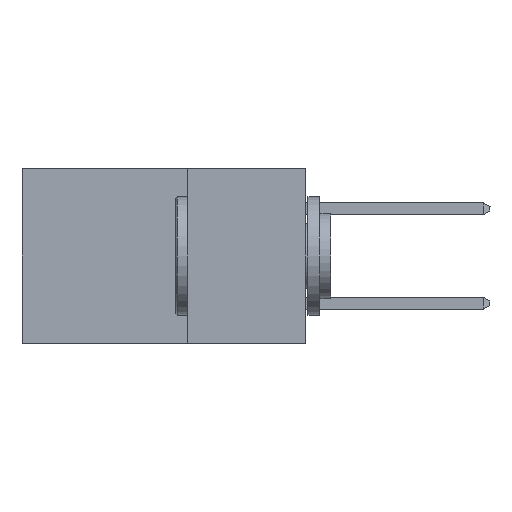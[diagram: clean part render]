
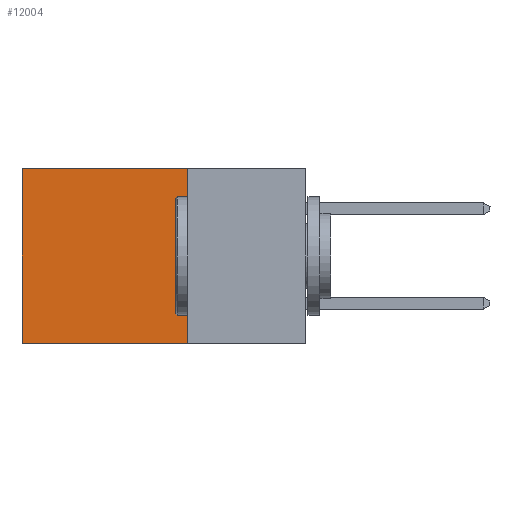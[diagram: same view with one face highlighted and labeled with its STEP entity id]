
A CAD part, left-side view. The second image highlights one B-rep face of the part: STEP entity #12004.
In plain terms, the highlighted planar face has unit normal (-1, 0, 0).
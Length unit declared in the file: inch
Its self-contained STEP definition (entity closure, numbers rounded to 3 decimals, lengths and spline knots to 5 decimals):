
#1661 = AXIS2_PLACEMENT_3D ( 'NONE', #18936, #21601, #6206 ) ;
#2513 = EDGE_CURVE ( 'NONE', #15147, #22574, #18310, .T. ) ;
#3587 = PLANE ( 'NONE',  #1661 ) ;
#4843 = EDGE_LOOP ( 'NONE', ( #19718, #20864, #5528, #10257 ) ) ;
#5085 = CARTESIAN_POINT ( 'NONE',  ( 0.298, 0.25, 0. ) ) ;
#5528 = ORIENTED_EDGE ( 'NONE', *, *, #19236, .F. ) ;
#5930 = LINE ( 'NONE', #11787, #24842 ) ;
#6206 = DIRECTION ( 'NONE',  ( 0., 0., -1. ) ) ;
#6386 = VERTEX_POINT ( 'NONE', #13751 ) ;
#10257 = ORIENTED_EDGE ( 'NONE', *, *, #29645, .T. ) ;
#11787 = CARTESIAN_POINT ( 'NONE',  ( 0.298, 0.25, 0. ) ) ;
#12004 = ADVANCED_FACE ( 'NONE', ( #19740 ), #3587, .F. ) ;
#12208 = VECTOR ( 'NONE', #12736, 39.37008 ) ;
#12736 = DIRECTION ( 'NONE',  ( 0., 1., 0. ) ) ;
#13751 = CARTESIAN_POINT ( 'NONE',  ( 0.298, 0.25, -0.37 ) ) ;
#14471 = DIRECTION ( 'NONE',  ( 0., 0., -1. ) ) ;
#15147 = VERTEX_POINT ( 'NONE', #18187 ) ;
#15740 = EDGE_CURVE ( 'NONE', #6386, #22574, #18259, .T. ) ;
#16631 = LINE ( 'NONE', #32372, #23445 ) ;
#16966 = DIRECTION ( 'NONE',  ( 0., 1., 0. ) ) ;
#18187 = CARTESIAN_POINT ( 'NONE',  ( 0.298, 0.6, 0. ) ) ;
#18259 = LINE ( 'NONE', #28138, #12208 ) ;
#18310 = LINE ( 'NONE', #21488, #24311 ) ;
#18936 = CARTESIAN_POINT ( 'NONE',  ( 0.298, 0.25, 0. ) ) ;
#19236 = EDGE_CURVE ( 'NONE', #20137, #6386, #16631, .T. ) ;
#19718 = ORIENTED_EDGE ( 'NONE', *, *, #2513, .T. ) ;
#19740 = FACE_OUTER_BOUND ( 'NONE', #4843, .T. ) ;
#20137 = VERTEX_POINT ( 'NONE', #5085 ) ;
#20864 = ORIENTED_EDGE ( 'NONE', *, *, #15740, .F. ) ;
#21488 = CARTESIAN_POINT ( 'NONE',  ( 0.298, 0.6, 0. ) ) ;
#21601 = DIRECTION ( 'NONE',  ( 1., 0., 0. ) ) ;
#22574 = VERTEX_POINT ( 'NONE', #29902 ) ;
#23445 = VECTOR ( 'NONE', #14471, 39.37008 ) ;
#23572 = DIRECTION ( 'NONE',  ( 0., 0., -1. ) ) ;
#24311 = VECTOR ( 'NONE', #23572, 39.37008 ) ;
#24842 = VECTOR ( 'NONE', #16966, 39.37008 ) ;
#28138 = CARTESIAN_POINT ( 'NONE',  ( 0.298, 0.25, -0.37 ) ) ;
#29645 = EDGE_CURVE ( 'NONE', #20137, #15147, #5930, .T. ) ;
#29902 = CARTESIAN_POINT ( 'NONE',  ( 0.298, 0.6, -0.37 ) ) ;
#32372 = CARTESIAN_POINT ( 'NONE',  ( 0.298, 0.25, 0. ) ) ;
